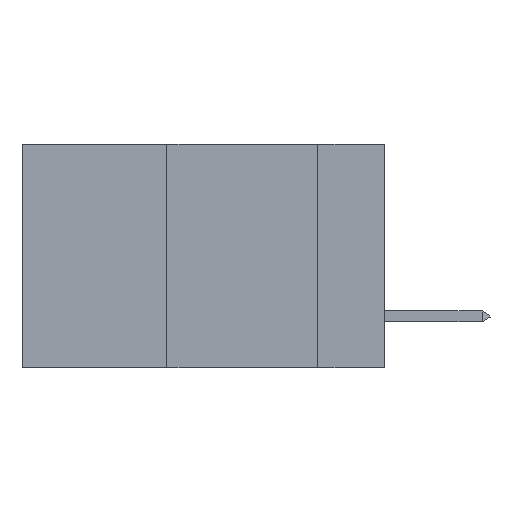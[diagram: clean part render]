
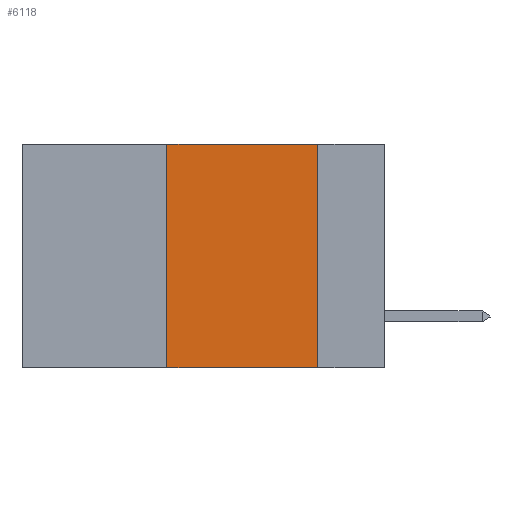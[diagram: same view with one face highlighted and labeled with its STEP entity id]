
A CAD part, left-side view. The second image highlights one B-rep face of the part: STEP entity #6118.
In plain terms, the highlighted planar face has unit normal (-1, 0, 0).
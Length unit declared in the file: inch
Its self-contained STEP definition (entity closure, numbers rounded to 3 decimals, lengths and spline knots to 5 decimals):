
#608 = LINE ( 'NONE', #5260, #8895 ) ;
#626 = FACE_OUTER_BOUND ( 'NONE', #3709, .T. ) ;
#1241 = LINE ( 'NONE', #11592, #4285 ) ;
#1346 = ORIENTED_EDGE ( 'NONE', *, *, #11482, .F. ) ;
#1524 = EDGE_CURVE ( 'NONE', #10133, #8385, #1241, .T. ) ;
#1694 = CARTESIAN_POINT ( 'NONE',  ( 0., 0.36, 0. ) ) ;
#2501 = DIRECTION ( 'NONE',  ( 0., -1., 0. ) ) ;
#2769 = DIRECTION ( 'NONE',  ( 0., -1., 0. ) ) ;
#2874 = CARTESIAN_POINT ( 'NONE',  ( 0., 0.11, -0.37 ) ) ;
#3412 = ORIENTED_EDGE ( 'NONE', *, *, #1524, .F. ) ;
#3658 = CARTESIAN_POINT ( 'NONE',  ( 0., 0.36, -0.37 ) ) ;
#3709 = EDGE_LOOP ( 'NONE', ( #4359, #1346, #3412, #8550 ) ) ;
#4234 = DIRECTION ( 'NONE',  ( 1., 0., 0. ) ) ;
#4249 = VERTEX_POINT ( 'NONE', #2874 ) ;
#4285 = VECTOR ( 'NONE', #4788, 39.37008 ) ;
#4359 = ORIENTED_EDGE ( 'NONE', *, *, #7765, .F. ) ;
#4782 = VECTOR ( 'NONE', #2769, 39.37008 ) ;
#4788 = DIRECTION ( 'NONE',  ( 0., 0., 1. ) ) ;
#5018 = AXIS2_PLACEMENT_3D ( 'NONE', #5167, #4234, #11890 ) ;
#5167 = CARTESIAN_POINT ( 'NONE',  ( 0., 0.6, 0. ) ) ;
#5184 = VECTOR ( 'NONE', #2501, 39.37008 ) ;
#5260 = CARTESIAN_POINT ( 'NONE',  ( 0., 0.11, 0. ) ) ;
#5793 = LINE ( 'NONE', #8353, #5184 ) ;
#6118 = ADVANCED_FACE ( 'NONE', ( #626 ), #7017, .F. ) ;
#6654 = CARTESIAN_POINT ( 'NONE',  ( 0., 0.6, 0. ) ) ;
#7017 = PLANE ( 'NONE',  #5018 ) ;
#7765 = EDGE_CURVE ( 'NONE', #10455, #4249, #608, .T. ) ;
#8179 = LINE ( 'NONE', #6654, #4782 ) ;
#8255 = EDGE_CURVE ( 'NONE', #10133, #4249, #5793, .T. ) ;
#8353 = CARTESIAN_POINT ( 'NONE',  ( 0., 0.6, -0.37 ) ) ;
#8385 = VERTEX_POINT ( 'NONE', #1694 ) ;
#8392 = CARTESIAN_POINT ( 'NONE',  ( 0., 0.11, 0. ) ) ;
#8550 = ORIENTED_EDGE ( 'NONE', *, *, #8255, .T. ) ;
#8895 = VECTOR ( 'NONE', #11042, 39.37008 ) ;
#10133 = VERTEX_POINT ( 'NONE', #3658 ) ;
#10455 = VERTEX_POINT ( 'NONE', #8392 ) ;
#11042 = DIRECTION ( 'NONE',  ( 0., 0., -1. ) ) ;
#11482 = EDGE_CURVE ( 'NONE', #8385, #10455, #8179, .T. ) ;
#11592 = CARTESIAN_POINT ( 'NONE',  ( 0., 0.36, 0. ) ) ;
#11890 = DIRECTION ( 'NONE',  ( 0., 0., -1. ) ) ;
